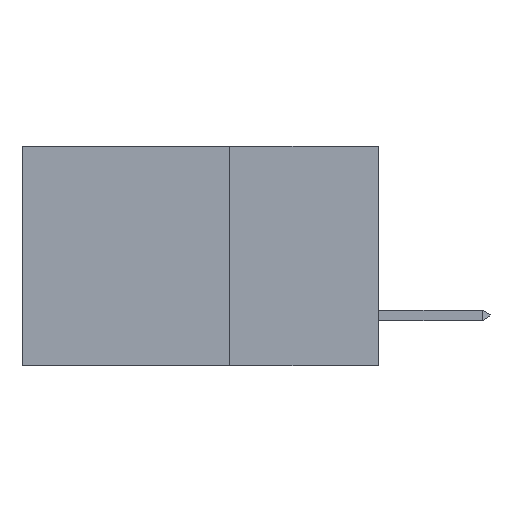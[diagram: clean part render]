
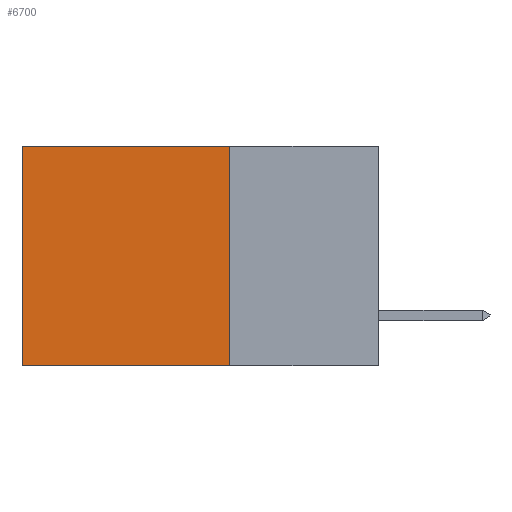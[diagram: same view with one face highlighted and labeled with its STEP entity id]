
A CAD part, left-side view. The second image highlights one B-rep face of the part: STEP entity #6700.
In plain terms, the highlighted planar face has unit normal (-1, 0, 0).
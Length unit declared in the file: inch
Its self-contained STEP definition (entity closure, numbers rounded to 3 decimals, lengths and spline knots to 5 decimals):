
#349 = EDGE_CURVE ( 'NONE', #1683, #1155, #8255, .T. ) ;
#523 = VECTOR ( 'NONE', #5258, 39.37008 ) ;
#1155 = VERTEX_POINT ( 'NONE', #15180 ) ;
#1683 = VERTEX_POINT ( 'NONE', #15292 ) ;
#2480 = EDGE_LOOP ( 'NONE', ( #5841, #7910, #3447, #7352 ) ) ;
#2612 = VECTOR ( 'NONE', #14705, 39.37008 ) ;
#2900 = DIRECTION ( 'NONE',  ( 0., 0., -1. ) ) ;
#3057 = CARTESIAN_POINT ( 'NONE',  ( 0.298, 0.25, 0. ) ) ;
#3447 = ORIENTED_EDGE ( 'NONE', *, *, #349, .F. ) ;
#3801 = LINE ( 'NONE', #16635, #15432 ) ;
#5249 = LINE ( 'NONE', #10678, #523 ) ;
#5258 = DIRECTION ( 'NONE',  ( 0., 1., 0. ) ) ;
#5801 = AXIS2_PLACEMENT_3D ( 'NONE', #6950, #13636, #2900 ) ;
#5841 = ORIENTED_EDGE ( 'NONE', *, *, #11722, .T. ) ;
#6437 = DIRECTION ( 'NONE',  ( 0., 1., 0. ) ) ;
#6700 = ADVANCED_FACE ( 'NONE', ( #11948 ), #9597, .F. ) ;
#6950 = CARTESIAN_POINT ( 'NONE',  ( 0.298, 0.25, 0. ) ) ;
#7352 = ORIENTED_EDGE ( 'NONE', *, *, #10878, .T. ) ;
#7489 = EDGE_CURVE ( 'NONE', #1155, #11604, #5249, .T. ) ;
#7910 = ORIENTED_EDGE ( 'NONE', *, *, #7489, .F. ) ;
#8255 = LINE ( 'NONE', #14937, #2612 ) ;
#9597 = PLANE ( 'NONE',  #5801 ) ;
#9833 = VERTEX_POINT ( 'NONE', #12739 ) ;
#10678 = CARTESIAN_POINT ( 'NONE',  ( 0.298, 0.25, -0.37 ) ) ;
#10878 = EDGE_CURVE ( 'NONE', #1683, #9833, #12557, .T. ) ;
#11604 = VERTEX_POINT ( 'NONE', #16399 ) ;
#11722 = EDGE_CURVE ( 'NONE', #9833, #11604, #3801, .T. ) ;
#11948 = FACE_OUTER_BOUND ( 'NONE', #2480, .T. ) ;
#12546 = DIRECTION ( 'NONE',  ( 0., 0., -1. ) ) ;
#12557 = LINE ( 'NONE', #3057, #15906 ) ;
#12739 = CARTESIAN_POINT ( 'NONE',  ( 0.298, 0.6, 0. ) ) ;
#13636 = DIRECTION ( 'NONE',  ( 1., 0., 0. ) ) ;
#14705 = DIRECTION ( 'NONE',  ( 0., 0., -1. ) ) ;
#14937 = CARTESIAN_POINT ( 'NONE',  ( 0.298, 0.25, 0. ) ) ;
#15180 = CARTESIAN_POINT ( 'NONE',  ( 0.298, 0.25, -0.37 ) ) ;
#15292 = CARTESIAN_POINT ( 'NONE',  ( 0.298, 0.25, 0. ) ) ;
#15432 = VECTOR ( 'NONE', #12546, 39.37008 ) ;
#15906 = VECTOR ( 'NONE', #6437, 39.37008 ) ;
#16399 = CARTESIAN_POINT ( 'NONE',  ( 0.298, 0.6, -0.37 ) ) ;
#16635 = CARTESIAN_POINT ( 'NONE',  ( 0.298, 0.6, 0. ) ) ;
